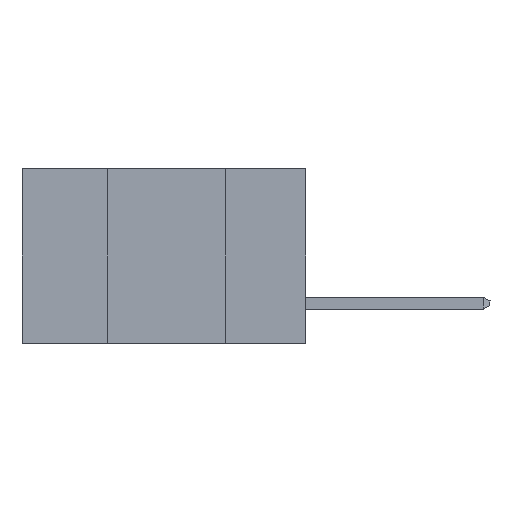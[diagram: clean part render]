
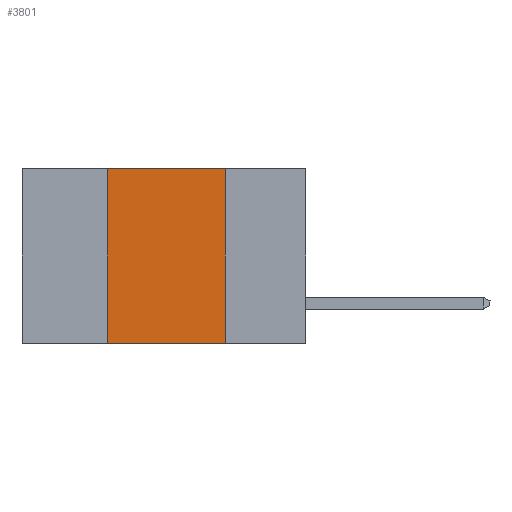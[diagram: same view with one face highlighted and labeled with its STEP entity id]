
A CAD part, left-side view. The second image highlights one B-rep face of the part: STEP entity #3801.
In plain terms, the highlighted planar face has unit normal (-1, 0, 0).
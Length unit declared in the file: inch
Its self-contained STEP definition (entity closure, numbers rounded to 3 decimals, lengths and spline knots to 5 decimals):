
#1467 = EDGE_LOOP ( 'NONE', ( #14525, #4295, #17470, #17205 ) ) ;
#1921 = CARTESIAN_POINT ( 'NONE',  ( 0., 0.17, 0. ) ) ;
#3498 = FACE_OUTER_BOUND ( 'NONE', #1467, .T. ) ;
#3801 = ADVANCED_FACE ( 'NONE', ( #3498 ), #17069, .F. ) ;
#4295 = ORIENTED_EDGE ( 'NONE', *, *, #17222, .F. ) ;
#4581 = EDGE_CURVE ( 'NONE', #11209, #18031, #12190, .T. ) ;
#5334 = DIRECTION ( 'NONE',  ( 0., 0., -1. ) ) ;
#5466 = DIRECTION ( 'NONE',  ( 1., 0., 0. ) ) ;
#5468 = CARTESIAN_POINT ( 'NONE',  ( 0., 0.42, -0.37 ) ) ;
#6427 = DIRECTION ( 'NONE',  ( 0., 0., 1. ) ) ;
#6776 = CARTESIAN_POINT ( 'NONE',  ( 0., 0.17, 0. ) ) ;
#6879 = VERTEX_POINT ( 'NONE', #19040 ) ;
#7305 = LINE ( 'NONE', #16559, #9817 ) ;
#7665 = DIRECTION ( 'NONE',  ( 0., -1., 0. ) ) ;
#9817 = VECTOR ( 'NONE', #6427, 39.37008 ) ;
#9852 = LINE ( 'NONE', #1921, #14921 ) ;
#10557 = CARTESIAN_POINT ( 'NONE',  ( 0., 0.6, 0. ) ) ;
#11095 = CARTESIAN_POINT ( 'NONE',  ( 0., 0.17, -0.37 ) ) ;
#11209 = VERTEX_POINT ( 'NONE', #5468 ) ;
#11356 = CARTESIAN_POINT ( 'NONE',  ( 0., 0.6, -0.37 ) ) ;
#11710 = LINE ( 'NONE', #10557, #12875 ) ;
#11986 = VECTOR ( 'NONE', #11998, 39.37008 ) ;
#11998 = DIRECTION ( 'NONE',  ( 0., -1., 0. ) ) ;
#12190 = LINE ( 'NONE', #11356, #11986 ) ;
#12875 = VECTOR ( 'NONE', #7665, 39.37008 ) ;
#13461 = DIRECTION ( 'NONE',  ( 0., 0., -1. ) ) ;
#14238 = CARTESIAN_POINT ( 'NONE',  ( 0., 0.6, 0. ) ) ;
#14525 = ORIENTED_EDGE ( 'NONE', *, *, #17275, .F. ) ;
#14793 = AXIS2_PLACEMENT_3D ( 'NONE', #14238, #5466, #5334 ) ;
#14921 = VECTOR ( 'NONE', #13461, 39.37008 ) ;
#15080 = VERTEX_POINT ( 'NONE', #6776 ) ;
#16559 = CARTESIAN_POINT ( 'NONE',  ( 0., 0.42, 0. ) ) ;
#17069 = PLANE ( 'NONE',  #14793 ) ;
#17205 = ORIENTED_EDGE ( 'NONE', *, *, #4581, .T. ) ;
#17222 = EDGE_CURVE ( 'NONE', #6879, #15080, #11710, .T. ) ;
#17275 = EDGE_CURVE ( 'NONE', #15080, #18031, #9852, .T. ) ;
#17470 = ORIENTED_EDGE ( 'NONE', *, *, #18017, .F. ) ;
#18017 = EDGE_CURVE ( 'NONE', #11209, #6879, #7305, .T. ) ;
#18031 = VERTEX_POINT ( 'NONE', #11095 ) ;
#19040 = CARTESIAN_POINT ( 'NONE',  ( 0., 0.42, 0. ) ) ;
